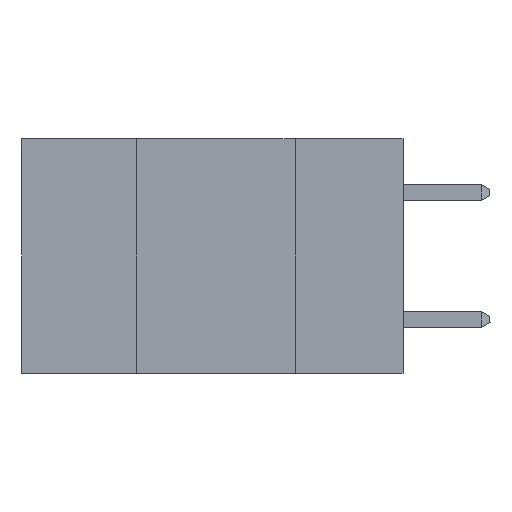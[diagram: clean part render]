
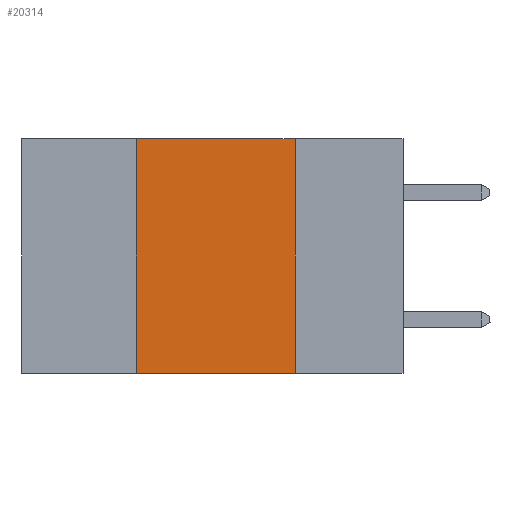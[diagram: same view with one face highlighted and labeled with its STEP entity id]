
A CAD part, left-side view. The second image highlights one B-rep face of the part: STEP entity #20314.
In plain terms, the highlighted planar face has unit normal (-1, 0, 0).
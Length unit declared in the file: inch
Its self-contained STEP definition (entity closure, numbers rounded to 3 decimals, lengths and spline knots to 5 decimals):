
#157 = EDGE_CURVE ( 'NONE', #6769, #20410, #25793, .T. ) ;
#1351 = CARTESIAN_POINT ( 'NONE',  ( 0., 0.17, -0.37 ) ) ;
#1446 = DIRECTION ( 'NONE',  ( 0., -1., 0. ) ) ;
#3007 = ORIENTED_EDGE ( 'NONE', *, *, #157, .F. ) ;
#3584 = LINE ( 'NONE', #22417, #13614 ) ;
#4857 = VECTOR ( 'NONE', #16575, 39.37008 ) ;
#4921 = CARTESIAN_POINT ( 'NONE',  ( 0., 0.6, 0. ) ) ;
#6769 = VERTEX_POINT ( 'NONE', #15472 ) ;
#6808 = FACE_OUTER_BOUND ( 'NONE', #21374, .T. ) ;
#7130 = PLANE ( 'NONE',  #12311 ) ;
#7136 = CARTESIAN_POINT ( 'NONE',  ( 0., 0.6, -0.37 ) ) ;
#7666 = VECTOR ( 'NONE', #16869, 39.37008 ) ;
#8782 = DIRECTION ( 'NONE',  ( 0., 0., -1. ) ) ;
#11038 = CARTESIAN_POINT ( 'NONE',  ( 0., 0.6, 0. ) ) ;
#11570 = CARTESIAN_POINT ( 'NONE',  ( 0., 0.17, 0. ) ) ;
#12311 = AXIS2_PLACEMENT_3D ( 'NONE', #4921, #16983, #12909 ) ;
#12909 = DIRECTION ( 'NONE',  ( 0., 0., -1. ) ) ;
#13241 = EDGE_CURVE ( 'NONE', #20410, #15711, #3584, .T. ) ;
#13614 = VECTOR ( 'NONE', #8782, 39.37008 ) ;
#15472 = CARTESIAN_POINT ( 'NONE',  ( 0., 0.42, 0. ) ) ;
#15711 = VERTEX_POINT ( 'NONE', #1351 ) ;
#16575 = DIRECTION ( 'NONE',  ( 0., 0., 1. ) ) ;
#16869 = DIRECTION ( 'NONE',  ( 0., -1., 0. ) ) ;
#16983 = DIRECTION ( 'NONE',  ( 1., 0., 0. ) ) ;
#17378 = LINE ( 'NONE', #24812, #4857 ) ;
#17578 = EDGE_CURVE ( 'NONE', #21164, #15711, #18391, .T. ) ;
#17826 = ORIENTED_EDGE ( 'NONE', *, *, #25402, .F. ) ;
#18391 = LINE ( 'NONE', #7136, #22493 ) ;
#19625 = ORIENTED_EDGE ( 'NONE', *, *, #17578, .T. ) ;
#20314 = ADVANCED_FACE ( 'NONE', ( #6808 ), #7130, .F. ) ;
#20410 = VERTEX_POINT ( 'NONE', #11570 ) ;
#21164 = VERTEX_POINT ( 'NONE', #23427 ) ;
#21374 = EDGE_LOOP ( 'NONE', ( #23217, #3007, #17826, #19625 ) ) ;
#22417 = CARTESIAN_POINT ( 'NONE',  ( 0., 0.17, 0. ) ) ;
#22493 = VECTOR ( 'NONE', #1446, 39.37008 ) ;
#23217 = ORIENTED_EDGE ( 'NONE', *, *, #13241, .F. ) ;
#23427 = CARTESIAN_POINT ( 'NONE',  ( 0., 0.42, -0.37 ) ) ;
#24812 = CARTESIAN_POINT ( 'NONE',  ( 0., 0.42, 0. ) ) ;
#25402 = EDGE_CURVE ( 'NONE', #21164, #6769, #17378, .T. ) ;
#25793 = LINE ( 'NONE', #11038, #7666 ) ;
